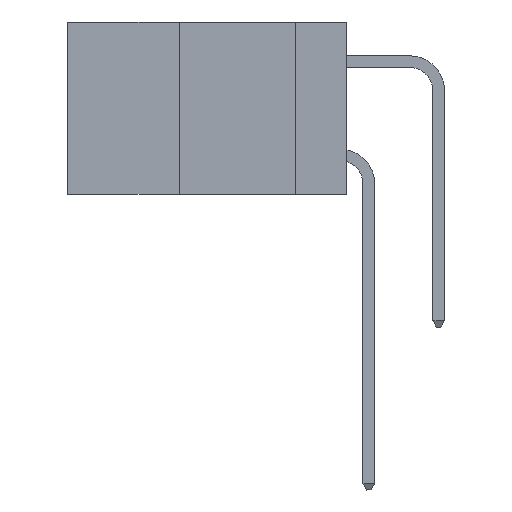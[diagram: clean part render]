
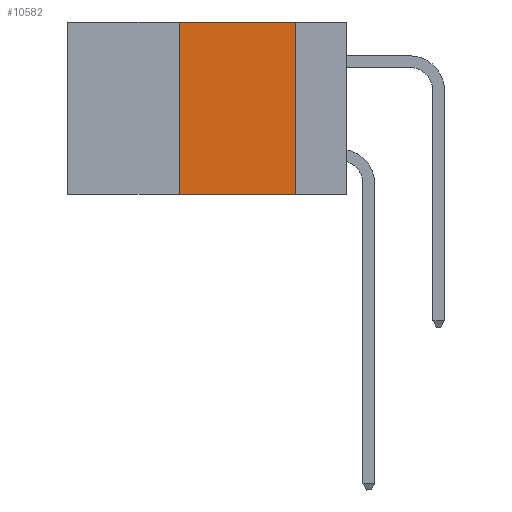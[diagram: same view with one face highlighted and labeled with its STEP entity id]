
A CAD part, left-side view. The second image highlights one B-rep face of the part: STEP entity #10582.
In plain terms, the highlighted planar face has unit normal (-1, 0, 0).
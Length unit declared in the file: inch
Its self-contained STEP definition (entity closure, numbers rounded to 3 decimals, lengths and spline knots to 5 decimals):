
#137 = CARTESIAN_POINT ( 'NONE',  ( 0., 0.36, 0. ) ) ;
#509 = VERTEX_POINT ( 'NONE', #15054 ) ;
#565 = VERTEX_POINT ( 'NONE', #4968 ) ;
#1315 = CARTESIAN_POINT ( 'NONE',  ( 0., 0.11, 0. ) ) ;
#1395 = DIRECTION ( 'NONE',  ( 0., -1., 0. ) ) ;
#1771 = VERTEX_POINT ( 'NONE', #26398 ) ;
#2304 = VECTOR ( 'NONE', #1395, 39.37008 ) ;
#3512 = DIRECTION ( 'NONE',  ( 0., 0., -1. ) ) ;
#3527 = EDGE_CURVE ( 'NONE', #565, #1771, #4440, .T. ) ;
#3729 = DIRECTION ( 'NONE',  ( 0., -1., 0. ) ) ;
#3784 = CARTESIAN_POINT ( 'NONE',  ( 0., 0.6, 0. ) ) ;
#4440 = LINE ( 'NONE', #1315, #5132 ) ;
#4968 = CARTESIAN_POINT ( 'NONE',  ( 0., 0.11, 0. ) ) ;
#5132 = VECTOR ( 'NONE', #3512, 39.37008 ) ;
#5655 = LINE ( 'NONE', #12383, #15697 ) ;
#6544 = LINE ( 'NONE', #137, #16543 ) ;
#6659 = DIRECTION ( 'NONE',  ( 0., 0., 1. ) ) ;
#7156 = FACE_OUTER_BOUND ( 'NONE', #8175, .T. ) ;
#7422 = EDGE_CURVE ( 'NONE', #509, #1771, #5655, .T. ) ;
#8175 = EDGE_LOOP ( 'NONE', ( #26659, #27314, #16937, #23150 ) ) ;
#8201 = DIRECTION ( 'NONE',  ( 0., 0., -1. ) ) ;
#10582 = ADVANCED_FACE ( 'NONE', ( #7156 ), #18779, .F. ) ;
#12246 = CARTESIAN_POINT ( 'NONE',  ( 0., 0.6, 0. ) ) ;
#12296 = CARTESIAN_POINT ( 'NONE',  ( 0., 0.36, 0. ) ) ;
#12383 = CARTESIAN_POINT ( 'NONE',  ( 0., 0.6, -0.37 ) ) ;
#15054 = CARTESIAN_POINT ( 'NONE',  ( 0., 0.36, -0.37 ) ) ;
#15697 = VECTOR ( 'NONE', #3729, 39.37008 ) ;
#16543 = VECTOR ( 'NONE', #6659, 39.37008 ) ;
#16556 = EDGE_CURVE ( 'NONE', #509, #26785, #6544, .T. ) ;
#16937 = ORIENTED_EDGE ( 'NONE', *, *, #16556, .F. ) ;
#18779 = PLANE ( 'NONE',  #25545 ) ;
#20862 = DIRECTION ( 'NONE',  ( 1., 0., 0. ) ) ;
#23150 = ORIENTED_EDGE ( 'NONE', *, *, #7422, .T. ) ;
#23903 = EDGE_CURVE ( 'NONE', #26785, #565, #24925, .T. ) ;
#24925 = LINE ( 'NONE', #12246, #2304 ) ;
#25545 = AXIS2_PLACEMENT_3D ( 'NONE', #3784, #20862, #8201 ) ;
#26398 = CARTESIAN_POINT ( 'NONE',  ( 0., 0.11, -0.37 ) ) ;
#26659 = ORIENTED_EDGE ( 'NONE', *, *, #3527, .F. ) ;
#26785 = VERTEX_POINT ( 'NONE', #12296 ) ;
#27314 = ORIENTED_EDGE ( 'NONE', *, *, #23903, .F. ) ;
